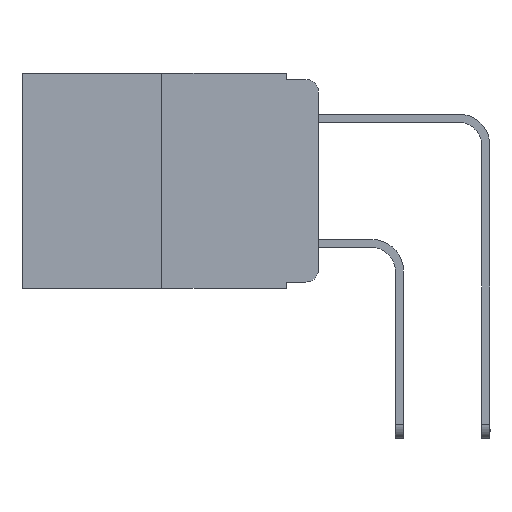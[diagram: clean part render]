
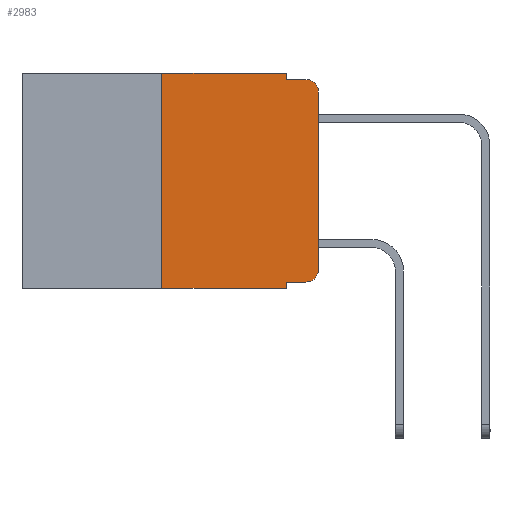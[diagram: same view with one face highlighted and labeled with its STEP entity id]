
A CAD part, left-side view. The second image highlights one B-rep face of the part: STEP entity #2983.
In plain terms, the highlighted planar face has unit normal (-1, 0, 0).
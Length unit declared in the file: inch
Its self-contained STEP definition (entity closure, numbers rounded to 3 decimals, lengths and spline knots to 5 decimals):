
#46 = VERTEX_POINT ( 'NONE', #1621 ) ;
#109 = CIRCLE ( 'NONE', #25644, 0.02 ) ;
#470 = VERTEX_POINT ( 'NONE', #11868 ) ;
#910 = CARTESIAN_POINT ( 'NONE',  ( 0., 0.051, 0. ) ) ;
#1417 = DIRECTION ( 'NONE',  ( 0., -1., 0. ) ) ;
#1491 = EDGE_CURVE ( 'NONE', #23667, #9689, #27236, .T. ) ;
#1621 = CARTESIAN_POINT ( 'NONE',  ( 0., 0.051, -0.333 ) ) ;
#1843 = ORIENTED_EDGE ( 'NONE', *, *, #15638, .F. ) ;
#2191 = LINE ( 'NONE', #10555, #11548 ) ;
#2504 = EDGE_LOOP ( 'NONE', ( #26309, #22776, #16618, #14768, #1843, #24470, #21087, #5745, #17298, #17440 ) ) ;
#2584 = EDGE_CURVE ( 'NONE', #470, #17172, #20681, .T. ) ;
#2700 = LINE ( 'NONE', #13344, #8743 ) ;
#2983 = ADVANCED_FACE ( 'NONE', ( #12952 ), #11878, .F. ) ;
#3131 = CARTESIAN_POINT ( 'NONE',  ( 0., 0.02, -0.01 ) ) ;
#3188 = CARTESIAN_POINT ( 'NONE',  ( 0., 0.473, 0. ) ) ;
#3320 = LINE ( 'NONE', #13832, #26767 ) ;
#4208 = VERTEX_POINT ( 'NONE', #6761 ) ;
#4708 = DIRECTION ( 'NONE',  ( 0., -1., 0. ) ) ;
#5064 = CARTESIAN_POINT ( 'NONE',  ( 0., 0.051, -0.343 ) ) ;
#5116 = EDGE_CURVE ( 'NONE', #46, #14709, #12891, .T. ) ;
#5745 = ORIENTED_EDGE ( 'NONE', *, *, #5116, .F. ) ;
#5754 = CARTESIAN_POINT ( 'NONE',  ( 0., 0.051, 0. ) ) ;
#6761 = CARTESIAN_POINT ( 'NONE',  ( 0., 0.25, 0. ) ) ;
#7391 = DIRECTION ( 'NONE',  ( 0., 0., -1. ) ) ;
#8743 = VECTOR ( 'NONE', #18023, 39.37008 ) ;
#9689 = VERTEX_POINT ( 'NONE', #22070 ) ;
#10167 = EDGE_CURVE ( 'NONE', #46, #23667, #2700, .T. ) ;
#10555 = CARTESIAN_POINT ( 'NONE',  ( 0., 0.473, 0. ) ) ;
#10578 = VECTOR ( 'NONE', #7391, 39.37008 ) ;
#11304 = CARTESIAN_POINT ( 'NONE',  ( 0., 0.02, -0.333 ) ) ;
#11548 = VECTOR ( 'NONE', #17105, 39.37008 ) ;
#11644 = CARTESIAN_POINT ( 'NONE',  ( 0., 0., -0.03 ) ) ;
#11868 = CARTESIAN_POINT ( 'NONE',  ( 0., 0.051, 0. ) ) ;
#11878 = PLANE ( 'NONE',  #17381 ) ;
#12442 = DIRECTION ( 'NONE',  ( -1., 0., 0. ) ) ;
#12891 = LINE ( 'NONE', #910, #10578 ) ;
#12952 = FACE_OUTER_BOUND ( 'NONE', #2504, .T. ) ;
#13074 = VERTEX_POINT ( 'NONE', #24130 ) ;
#13344 = CARTESIAN_POINT ( 'NONE',  ( 0., 0.051, -0.333 ) ) ;
#13832 = CARTESIAN_POINT ( 'NONE',  ( 0., 0., 0. ) ) ;
#13861 = DIRECTION ( 'NONE',  ( 1., 0., 0. ) ) ;
#14660 = AXIS2_PLACEMENT_3D ( 'NONE', #17283, #15215, #19670 ) ;
#14709 = VERTEX_POINT ( 'NONE', #5064 ) ;
#14768 = ORIENTED_EDGE ( 'NONE', *, *, #2584, .F. ) ;
#14781 = VECTOR ( 'NONE', #17254, 39.37008 ) ;
#15215 = DIRECTION ( 'NONE',  ( -1., 0., 0. ) ) ;
#15315 = VERTEX_POINT ( 'NONE', #11644 ) ;
#15338 = VECTOR ( 'NONE', #16413, 39.37008 ) ;
#15638 = EDGE_CURVE ( 'NONE', #4208, #470, #2191, .T. ) ;
#16024 = DIRECTION ( 'NONE',  ( 0., 0., -1. ) ) ;
#16343 = EDGE_CURVE ( 'NONE', #17172, #25777, #27596, .T. ) ;
#16413 = DIRECTION ( 'NONE',  ( 0., 0., -1. ) ) ;
#16618 = ORIENTED_EDGE ( 'NONE', *, *, #16343, .F. ) ;
#16740 = EDGE_CURVE ( 'NONE', #15315, #25777, #109, .T. ) ;
#17105 = DIRECTION ( 'NONE',  ( 0., -1., 0. ) ) ;
#17172 = VERTEX_POINT ( 'NONE', #18218 ) ;
#17254 = DIRECTION ( 'NONE',  ( 0., 0., 1. ) ) ;
#17283 = CARTESIAN_POINT ( 'NONE',  ( 0., 0.02, -0.313 ) ) ;
#17298 = ORIENTED_EDGE ( 'NONE', *, *, #10167, .T. ) ;
#17381 = AXIS2_PLACEMENT_3D ( 'NONE', #3188, #13861, #16024 ) ;
#17440 = ORIENTED_EDGE ( 'NONE', *, *, #1491, .T. ) ;
#17778 = VECTOR ( 'NONE', #1417, 39.37008 ) ;
#17895 = VECTOR ( 'NONE', #4708, 39.37008 ) ;
#18023 = DIRECTION ( 'NONE',  ( 0., -1., 0. ) ) ;
#18218 = CARTESIAN_POINT ( 'NONE',  ( 0., 0.051, -0.01 ) ) ;
#18996 = DIRECTION ( 'NONE',  ( 0., 0., -1. ) ) ;
#19129 = LINE ( 'NONE', #27058, #17778 ) ;
#19212 = CARTESIAN_POINT ( 'NONE',  ( 0., 0.25, 0. ) ) ;
#19670 = DIRECTION ( 'NONE',  ( 0., 0., -1. ) ) ;
#20681 = LINE ( 'NONE', #5754, #15338 ) ;
#21087 = ORIENTED_EDGE ( 'NONE', *, *, #22058, .T. ) ;
#21456 = LINE ( 'NONE', #19212, #14781 ) ;
#22058 = EDGE_CURVE ( 'NONE', #13074, #14709, #19129, .T. ) ;
#22070 = CARTESIAN_POINT ( 'NONE',  ( 0., 0., -0.313 ) ) ;
#22256 = EDGE_CURVE ( 'NONE', #13074, #4208, #21456, .T. ) ;
#22776 = ORIENTED_EDGE ( 'NONE', *, *, #16740, .T. ) ;
#23135 = CARTESIAN_POINT ( 'NONE',  ( 0., 0.02, -0.03 ) ) ;
#23667 = VERTEX_POINT ( 'NONE', #11304 ) ;
#23940 = DIRECTION ( 'NONE',  ( 0., 0., 1. ) ) ;
#24050 = CARTESIAN_POINT ( 'NONE',  ( 0., 0.051, -0.01 ) ) ;
#24130 = CARTESIAN_POINT ( 'NONE',  ( 0., 0.25, -0.343 ) ) ;
#24470 = ORIENTED_EDGE ( 'NONE', *, *, #22256, .F. ) ;
#25065 = EDGE_CURVE ( 'NONE', #9689, #15315, #3320, .T. ) ;
#25644 = AXIS2_PLACEMENT_3D ( 'NONE', #23135, #12442, #18996 ) ;
#25777 = VERTEX_POINT ( 'NONE', #3131 ) ;
#26309 = ORIENTED_EDGE ( 'NONE', *, *, #25065, .T. ) ;
#26767 = VECTOR ( 'NONE', #23940, 39.37008 ) ;
#27058 = CARTESIAN_POINT ( 'NONE',  ( 0., 0.473, -0.343 ) ) ;
#27236 = CIRCLE ( 'NONE', #14660, 0.02 ) ;
#27596 = LINE ( 'NONE', #24050, #17895 ) ;
